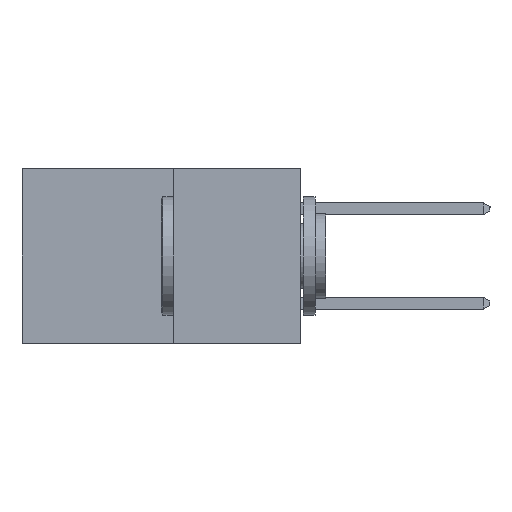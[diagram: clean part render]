
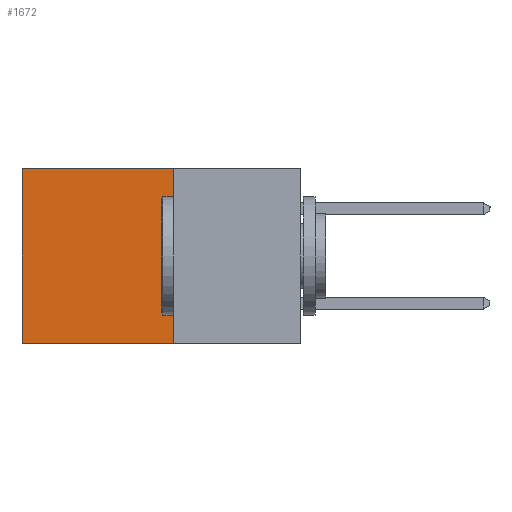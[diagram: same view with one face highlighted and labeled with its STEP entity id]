
A CAD part, left-side view. The second image highlights one B-rep face of the part: STEP entity #1672.
In plain terms, the highlighted planar face has unit normal (-1, 0, 0).
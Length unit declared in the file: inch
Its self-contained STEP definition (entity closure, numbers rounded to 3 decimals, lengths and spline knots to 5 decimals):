
#42 = CARTESIAN_POINT ( 'NONE',  ( 0.277, 0.27, -0.37 ) ) ;
#375 = DIRECTION ( 'NONE',  ( 0., 0., -1. ) ) ;
#463 = DIRECTION ( 'NONE',  ( 0., 0., -1. ) ) ;
#608 = VERTEX_POINT ( 'NONE', #6598 ) ;
#880 = EDGE_LOOP ( 'NONE', ( #2737, #8434, #5767, #1488 ) ) ;
#897 = CARTESIAN_POINT ( 'NONE',  ( 0.277, 0.59, -0.37 ) ) ;
#1116 = DIRECTION ( 'NONE',  ( 1., 0., 0. ) ) ;
#1296 = VECTOR ( 'NONE', #3764, 39.37008 ) ;
#1488 = ORIENTED_EDGE ( 'NONE', *, *, #5483, .T. ) ;
#1672 = ADVANCED_FACE ( 'NONE', ( #7114 ), #5474, .F. ) ;
#1844 = CARTESIAN_POINT ( 'NONE',  ( 0.277, 0.27, -0.37 ) ) ;
#2737 = ORIENTED_EDGE ( 'NONE', *, *, #7838, .T. ) ;
#2851 = VERTEX_POINT ( 'NONE', #897 ) ;
#2891 = LINE ( 'NONE', #3687, #5002 ) ;
#3663 = DIRECTION ( 'NONE',  ( 0., 1., 0. ) ) ;
#3687 = CARTESIAN_POINT ( 'NONE',  ( 0.277, 0.27, -0.37 ) ) ;
#3764 = DIRECTION ( 'NONE',  ( 0., 0., -1. ) ) ;
#3795 = CARTESIAN_POINT ( 'NONE',  ( 0.277, 0.59, -0.37 ) ) ;
#4353 = CARTESIAN_POINT ( 'NONE',  ( 0.277, 0.59, 0. ) ) ;
#4570 = VERTEX_POINT ( 'NONE', #1844 ) ;
#4649 = EDGE_CURVE ( 'NONE', #608, #4570, #7991, .T. ) ;
#5002 = VECTOR ( 'NONE', #3663, 39.37008 ) ;
#5220 = LINE ( 'NONE', #3795, #1296 ) ;
#5448 = CARTESIAN_POINT ( 'NONE',  ( 0.277, 0.27, 0. ) ) ;
#5461 = DIRECTION ( 'NONE',  ( 0., 1., 0. ) ) ;
#5474 = PLANE ( 'NONE',  #8518 ) ;
#5483 = EDGE_CURVE ( 'NONE', #608, #5759, #7005, .T. ) ;
#5759 = VERTEX_POINT ( 'NONE', #4353 ) ;
#5767 = ORIENTED_EDGE ( 'NONE', *, *, #4649, .F. ) ;
#5873 = VECTOR ( 'NONE', #375, 39.37008 ) ;
#6598 = CARTESIAN_POINT ( 'NONE',  ( 0.277, 0.27, 0. ) ) ;
#6769 = VECTOR ( 'NONE', #5461, 39.37008 ) ;
#7005 = LINE ( 'NONE', #5448, #6769 ) ;
#7114 = FACE_OUTER_BOUND ( 'NONE', #880, .T. ) ;
#7597 = CARTESIAN_POINT ( 'NONE',  ( 0.277, 0.27, -0.37 ) ) ;
#7838 = EDGE_CURVE ( 'NONE', #5759, #2851, #5220, .T. ) ;
#7857 = EDGE_CURVE ( 'NONE', #4570, #2851, #2891, .T. ) ;
#7991 = LINE ( 'NONE', #7597, #5873 ) ;
#8434 = ORIENTED_EDGE ( 'NONE', *, *, #7857, .F. ) ;
#8518 = AXIS2_PLACEMENT_3D ( 'NONE', #42, #1116, #463 ) ;
